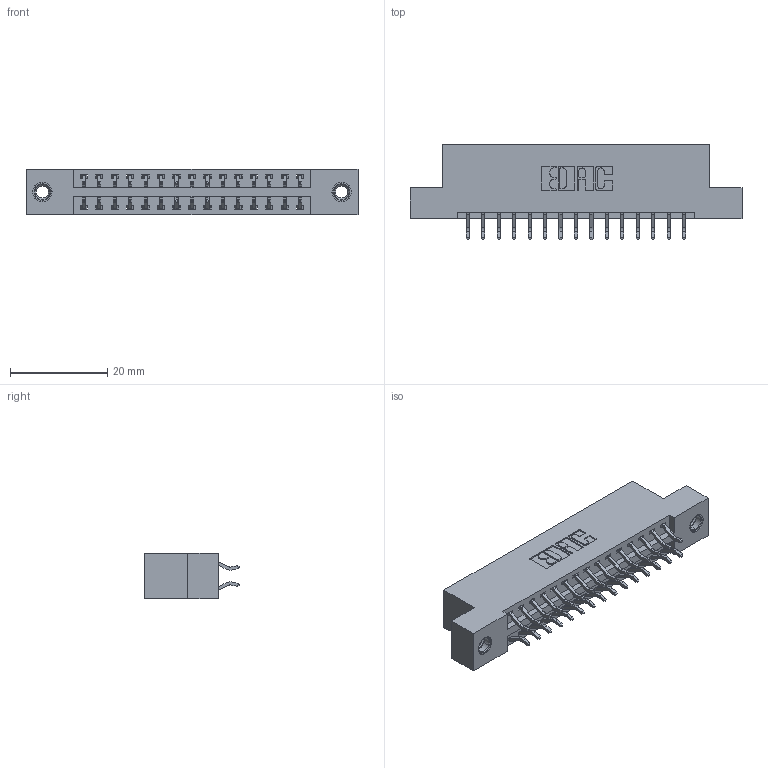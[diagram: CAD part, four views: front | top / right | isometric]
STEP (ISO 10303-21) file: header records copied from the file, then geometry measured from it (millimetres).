
FILE_DESCRIPTION (( 'STEP AP203' ), '1' );
FILE_NAME ('396-030-556-207.STEP', '2019-10-30T05:59:18', ( '' ), ( '' ), 'SwSTEP 2.0', 'SolidWorks 2016', '' );
FILE_SCHEMA (( 'CONFIG_CONTROL_DESIGN' ));
Length unit declared in the file: inch
Products named in the file (4): 345-250-001_345-250-005-103; 346 Part_Flush Mounting Lugs - 0.156 Dia-TI; 345-292-001_556 Tail; 396-030-556-207
Assembly tree (33 placements, depth 2):
  396-030-556-207
    346 Part_Flush Mounting Lugs - 0.156 Dia-TI
    345-292-001_556 Tail  x30
    345-250-001_345-250-005-103  x2
Bounding box: 68.2 x 19.57 x 9.4 mm (x, y, z)
Volume: 6425.8 mm3; surface area: 8414.3 mm2
Topology: 33 solids, 33 shells, 1922 faces, 5655 edges, 3722 vertices
Faces by surface type: plane 1278, cylinder 628, cone 12, torus 4
Entity records: 14830 total; most frequent: CARTESIAN_POINT 2479, ORIENTED_EDGE 2394, DIRECTION 2251, EDGE_CURVE 1197, LINE 977, VECTOR 977, VERTEX_POINT 792, AXIS2_PLACEMENT_3D 637
